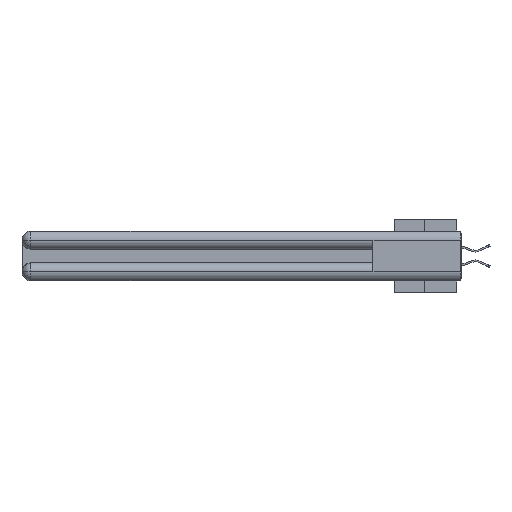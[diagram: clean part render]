
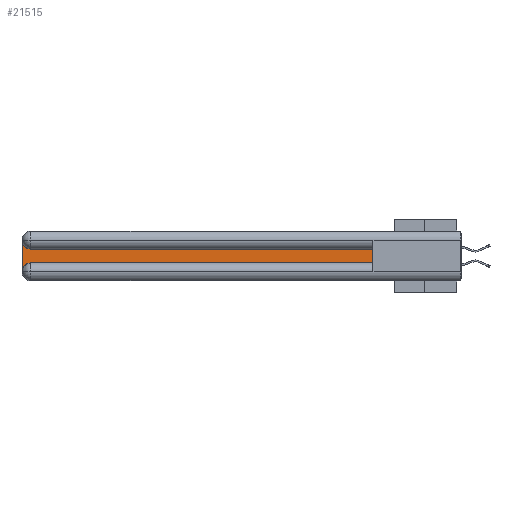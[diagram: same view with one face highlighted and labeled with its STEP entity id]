
A CAD part, left-side view. The second image highlights one B-rep face of the part: STEP entity #21515.
In plain terms, the highlighted planar face has unit normal (-1, 0, 0).
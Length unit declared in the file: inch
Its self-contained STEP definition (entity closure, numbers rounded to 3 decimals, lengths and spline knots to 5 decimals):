
#799 = LINE ( 'NONE', #11782, #9661 ) ;
#3362 = ORIENTED_EDGE ( 'NONE', *, *, #16983, .T. ) ;
#3424 = VECTOR ( 'NONE', #10752, 39.37008 ) ;
#6007 = CARTESIAN_POINT ( 'NONE',  ( 0.075, 2.94, -0.0625 ) ) ;
#8149 = VERTEX_POINT ( 'NONE', #35834 ) ;
#8300 = DIRECTION ( 'NONE',  ( 1., 0., 0. ) ) ;
#8738 = EDGE_LOOP ( 'NONE', ( #21209, #13316, #3362, #31978, #29615, #17606 ) ) ;
#8877 = FACE_OUTER_BOUND ( 'NONE', #8738, .T. ) ;
#9292 = CARTESIAN_POINT ( 'NONE',  ( 0.075, 2.94, -0.1225 ) ) ;
#9661 = VECTOR ( 'NONE', #36283, 39.37008 ) ;
#10260 = AXIS2_PLACEMENT_3D ( 'NONE', #6007, #8300, #12771 ) ;
#10589 = LINE ( 'NONE', #38770, #3424 ) ;
#10752 = DIRECTION ( 'NONE',  ( 0., 0., 1. ) ) ;
#11207 = CARTESIAN_POINT ( 'NONE',  ( 0.075, 2.94, -0.2175 ) ) ;
#11782 = CARTESIAN_POINT ( 'NONE',  ( 0.075, 3., -0.2175 ) ) ;
#12771 = DIRECTION ( 'NONE',  ( 0., 0., -1. ) ) ;
#12864 = PLANE ( 'NONE',  #25037 ) ;
#13316 = ORIENTED_EDGE ( 'NONE', *, *, #30073, .T. ) ;
#15370 = EDGE_CURVE ( 'NONE', #41773, #28659, #25147, .T. ) ;
#15825 = VECTOR ( 'NONE', #30472, 39.37008 ) ;
#15837 = CIRCLE ( 'NONE', #40419, 0.06 ) ;
#15883 = LINE ( 'NONE', #40388, #44953 ) ;
#16983 = EDGE_CURVE ( 'NONE', #28365, #42839, #799, .T. ) ;
#17606 = ORIENTED_EDGE ( 'NONE', *, *, #20835, .T. ) ;
#20080 = CARTESIAN_POINT ( 'NONE',  ( 0.075, 3., -0.1225 ) ) ;
#20835 = EDGE_CURVE ( 'NONE', #8149, #41773, #10589, .T. ) ;
#21087 = CARTESIAN_POINT ( 'NONE',  ( 0.075, 0.6, -0.1225 ) ) ;
#21209 = ORIENTED_EDGE ( 'NONE', *, *, #15370, .T. ) ;
#21515 = ADVANCED_FACE ( 'NONE', ( #8877 ), #12864, .F. ) ;
#22679 = CARTESIAN_POINT ( 'NONE',  ( 0.075, 3., -0.0625 ) ) ;
#23508 = CARTESIAN_POINT ( 'NONE',  ( 0.075, 3., -0.2775 ) ) ;
#23914 = DIRECTION ( 'NONE',  ( 1., 0., 0. ) ) ;
#24349 = CARTESIAN_POINT ( 'NONE',  ( 0.075, 2.94, -0.2775 ) ) ;
#24742 = CIRCLE ( 'NONE', #10260, 0.06 ) ;
#25037 = AXIS2_PLACEMENT_3D ( 'NONE', #20080, #37378, #34030 ) ;
#25147 = LINE ( 'NONE', #27096, #15825 ) ;
#27096 = CARTESIAN_POINT ( 'NONE',  ( 0.075, 0.6, -0.1225 ) ) ;
#28365 = VERTEX_POINT ( 'NONE', #22679 ) ;
#28659 = VERTEX_POINT ( 'NONE', #9292 ) ;
#29615 = ORIENTED_EDGE ( 'NONE', *, *, #38785, .T. ) ;
#30073 = EDGE_CURVE ( 'NONE', #28659, #28365, #24742, .T. ) ;
#30472 = DIRECTION ( 'NONE',  ( 0., 1., 0. ) ) ;
#31978 = ORIENTED_EDGE ( 'NONE', *, *, #36667, .T. ) ;
#34030 = DIRECTION ( 'NONE',  ( 0., 0., -1. ) ) ;
#34478 = DIRECTION ( 'NONE',  ( 0., 0., -1. ) ) ;
#35834 = CARTESIAN_POINT ( 'NONE',  ( 0.075, 0.6, -0.2175 ) ) ;
#35853 = VERTEX_POINT ( 'NONE', #11207 ) ;
#36283 = DIRECTION ( 'NONE',  ( 0., 0., -1. ) ) ;
#36667 = EDGE_CURVE ( 'NONE', #42839, #35853, #15837, .T. ) ;
#37378 = DIRECTION ( 'NONE',  ( 1., 0., 0. ) ) ;
#38770 = CARTESIAN_POINT ( 'NONE',  ( 0.075, 0.6, -0.2175 ) ) ;
#38785 = EDGE_CURVE ( 'NONE', #35853, #8149, #15883, .T. ) ;
#40388 = CARTESIAN_POINT ( 'NONE',  ( 0.075, 0.6, -0.2175 ) ) ;
#40419 = AXIS2_PLACEMENT_3D ( 'NONE', #24349, #23914, #34478 ) ;
#41773 = VERTEX_POINT ( 'NONE', #21087 ) ;
#42839 = VERTEX_POINT ( 'NONE', #23508 ) ;
#44039 = DIRECTION ( 'NONE',  ( 0., -1., 0. ) ) ;
#44953 = VECTOR ( 'NONE', #44039, 39.37008 ) ;
